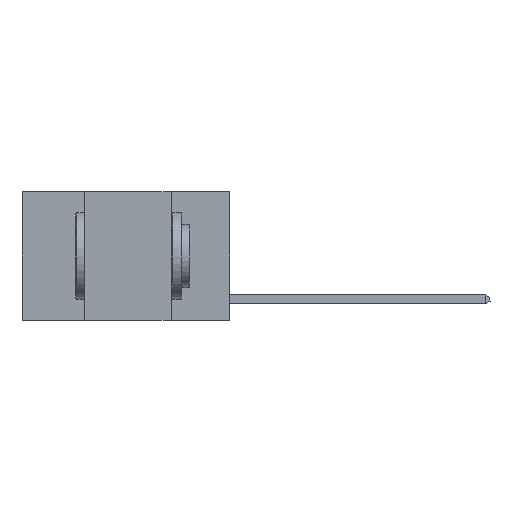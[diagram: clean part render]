
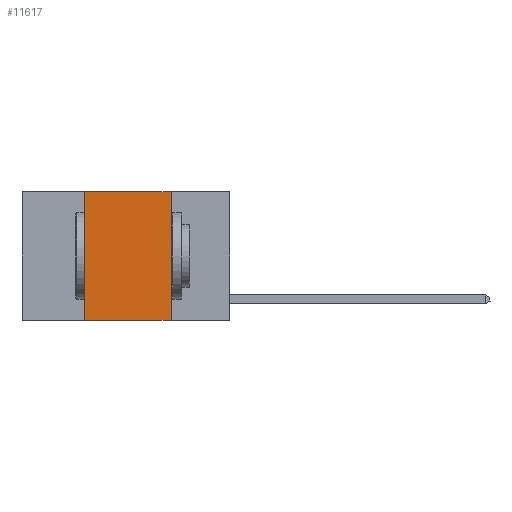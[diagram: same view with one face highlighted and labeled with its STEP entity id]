
A CAD part, left-side view. The second image highlights one B-rep face of the part: STEP entity #11617.
In plain terms, the highlighted planar face has unit normal (-1, 0, 0).
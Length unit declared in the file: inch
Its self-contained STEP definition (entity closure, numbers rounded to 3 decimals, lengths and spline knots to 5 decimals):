
#226 = LINE ( 'NONE', #2292, #7053 ) ;
#1514 = EDGE_CURVE ( 'NONE', #1920, #9731, #5209, .T. ) ;
#1920 = VERTEX_POINT ( 'NONE', #8053 ) ;
#2292 = CARTESIAN_POINT ( 'NONE',  ( 0., 0.6, 0. ) ) ;
#2578 = CARTESIAN_POINT ( 'NONE',  ( 0., 0.6, 0. ) ) ;
#2676 = EDGE_CURVE ( 'NONE', #1920, #11299, #2985, .T. ) ;
#2985 = LINE ( 'NONE', #9828, #10182 ) ;
#3232 = CARTESIAN_POINT ( 'NONE',  ( 0., 0.6, -0.37 ) ) ;
#3316 = VERTEX_POINT ( 'NONE', #4298 ) ;
#3544 = DIRECTION ( 'NONE',  ( 0., 0., -1. ) ) ;
#3758 = DIRECTION ( 'NONE',  ( 0., 0., 1. ) ) ;
#4298 = CARTESIAN_POINT ( 'NONE',  ( 0., 0.17, 0. ) ) ;
#5007 = CARTESIAN_POINT ( 'NONE',  ( 0., 0.42, 0. ) ) ;
#5209 = LINE ( 'NONE', #3232, #9540 ) ;
#5288 = DIRECTION ( 'NONE',  ( 0., -1., 0. ) ) ;
#5429 = EDGE_CURVE ( 'NONE', #11299, #3316, #226, .T. ) ;
#5774 = FACE_OUTER_BOUND ( 'NONE', #7248, .T. ) ;
#6345 = CARTESIAN_POINT ( 'NONE',  ( 0., 0.17, 0. ) ) ;
#6639 = VECTOR ( 'NONE', #3544, 39.37008 ) ;
#6820 = ORIENTED_EDGE ( 'NONE', *, *, #7221, .F. ) ;
#7053 = VECTOR ( 'NONE', #5288, 39.37008 ) ;
#7221 = EDGE_CURVE ( 'NONE', #3316, #9731, #12444, .T. ) ;
#7248 = EDGE_LOOP ( 'NONE', ( #6820, #11353, #10071, #10021 ) ) ;
#8053 = CARTESIAN_POINT ( 'NONE',  ( 0., 0.42, -0.37 ) ) ;
#8251 = DIRECTION ( 'NONE',  ( 0., -1., 0. ) ) ;
#8742 = AXIS2_PLACEMENT_3D ( 'NONE', #2578, #11527, #11659 ) ;
#9540 = VECTOR ( 'NONE', #8251, 39.37008 ) ;
#9731 = VERTEX_POINT ( 'NONE', #11412 ) ;
#9828 = CARTESIAN_POINT ( 'NONE',  ( 0., 0.42, 0. ) ) ;
#10021 = ORIENTED_EDGE ( 'NONE', *, *, #1514, .T. ) ;
#10071 = ORIENTED_EDGE ( 'NONE', *, *, #2676, .F. ) ;
#10182 = VECTOR ( 'NONE', #3758, 39.37008 ) ;
#11299 = VERTEX_POINT ( 'NONE', #5007 ) ;
#11353 = ORIENTED_EDGE ( 'NONE', *, *, #5429, .F. ) ;
#11412 = CARTESIAN_POINT ( 'NONE',  ( 0., 0.17, -0.37 ) ) ;
#11527 = DIRECTION ( 'NONE',  ( 1., 0., 0. ) ) ;
#11617 = ADVANCED_FACE ( 'NONE', ( #5774 ), #12422, .F. ) ;
#11659 = DIRECTION ( 'NONE',  ( 0., 0., -1. ) ) ;
#12422 = PLANE ( 'NONE',  #8742 ) ;
#12444 = LINE ( 'NONE', #6345, #6639 ) ;
